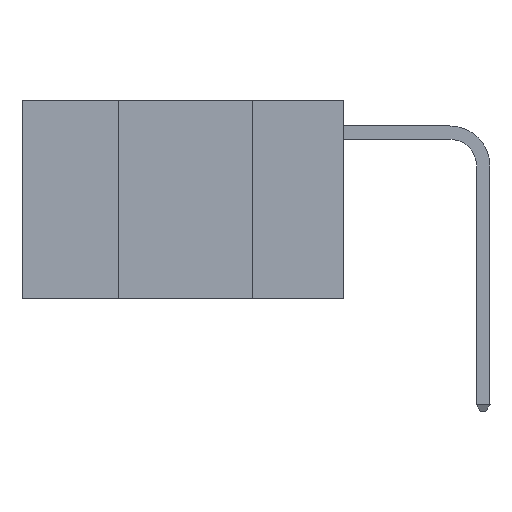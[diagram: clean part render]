
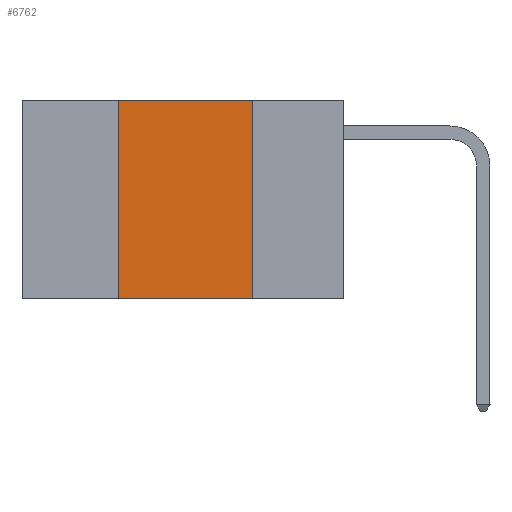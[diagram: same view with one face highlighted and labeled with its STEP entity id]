
A CAD part, left-side view. The second image highlights one B-rep face of the part: STEP entity #6762.
In plain terms, the highlighted planar face has unit normal (-1, 0, 0).
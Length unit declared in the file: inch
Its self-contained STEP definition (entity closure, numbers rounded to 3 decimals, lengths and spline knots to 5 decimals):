
#83 = LINE ( 'NONE', #457, #381 ) ;
#381 = VECTOR ( 'NONE', #482, 39.37008 ) ;
#457 = CARTESIAN_POINT ( 'NONE',  ( 0., 0.6, -0.37 ) ) ;
#482 = DIRECTION ( 'NONE',  ( 0., -1., 0. ) ) ;
#501 = DIRECTION ( 'NONE',  ( 0., -1., 0. ) ) ;
#814 = VECTOR ( 'NONE', #7738, 39.37008 ) ;
#915 = FACE_OUTER_BOUND ( 'NONE', #13519, .T. ) ;
#1237 = LINE ( 'NONE', #16533, #814 ) ;
#1289 = ORIENTED_EDGE ( 'NONE', *, *, #6891, .T. ) ;
#1367 = DIRECTION ( 'NONE',  ( 0., 0., -1. ) ) ;
#1374 = DIRECTION ( 'NONE',  ( 1., 0., 0. ) ) ;
#1432 = CARTESIAN_POINT ( 'NONE',  ( 0., 0.6, 0. ) ) ;
#1638 = EDGE_CURVE ( 'NONE', #16622, #3091, #16520, .T. ) ;
#1818 = PLANE ( 'NONE',  #10883 ) ;
#3091 = VERTEX_POINT ( 'NONE', #16362 ) ;
#4290 = VECTOR ( 'NONE', #16170, 39.37008 ) ;
#4562 = CARTESIAN_POINT ( 'NONE',  ( 0., 0.17, -0.37 ) ) ;
#6762 = ADVANCED_FACE ( 'NONE', ( #915 ), #1818, .F. ) ;
#6891 = EDGE_CURVE ( 'NONE', #13864, #12926, #83, .T. ) ;
#7369 = CARTESIAN_POINT ( 'NONE',  ( 0., 0.17, 0. ) ) ;
#7430 = LINE ( 'NONE', #7369, #4290 ) ;
#7738 = DIRECTION ( 'NONE',  ( 0., 0., 1. ) ) ;
#7984 = CARTESIAN_POINT ( 'NONE',  ( 0., 0.42, -0.37 ) ) ;
#8199 = ORIENTED_EDGE ( 'NONE', *, *, #11241, .F. ) ;
#9539 = EDGE_CURVE ( 'NONE', #13864, #16622, #1237, .T. ) ;
#10883 = AXIS2_PLACEMENT_3D ( 'NONE', #1432, #1374, #1367 ) ;
#11090 = ORIENTED_EDGE ( 'NONE', *, *, #1638, .F. ) ;
#11241 = EDGE_CURVE ( 'NONE', #3091, #12926, #7430, .T. ) ;
#12319 = CARTESIAN_POINT ( 'NONE',  ( 0., 0.6, 0. ) ) ;
#12926 = VERTEX_POINT ( 'NONE', #4562 ) ;
#13519 = EDGE_LOOP ( 'NONE', ( #8199, #11090, #15639, #1289 ) ) ;
#13864 = VERTEX_POINT ( 'NONE', #7984 ) ;
#15413 = CARTESIAN_POINT ( 'NONE',  ( 0., 0.42, 0. ) ) ;
#15639 = ORIENTED_EDGE ( 'NONE', *, *, #9539, .F. ) ;
#16170 = DIRECTION ( 'NONE',  ( 0., 0., -1. ) ) ;
#16249 = VECTOR ( 'NONE', #501, 39.37008 ) ;
#16362 = CARTESIAN_POINT ( 'NONE',  ( 0., 0.17, 0. ) ) ;
#16520 = LINE ( 'NONE', #12319, #16249 ) ;
#16533 = CARTESIAN_POINT ( 'NONE',  ( 0., 0.42, 0. ) ) ;
#16622 = VERTEX_POINT ( 'NONE', #15413 ) ;
